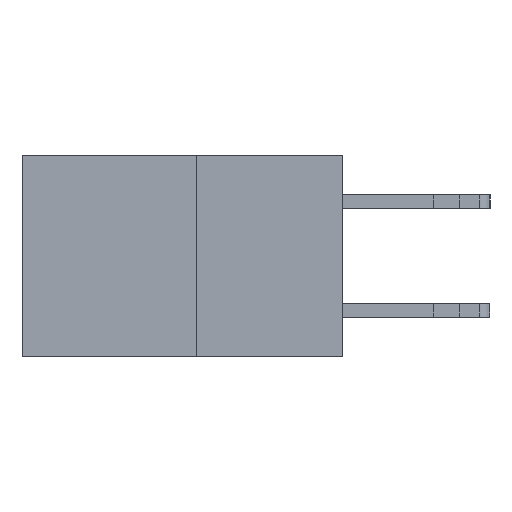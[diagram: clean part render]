
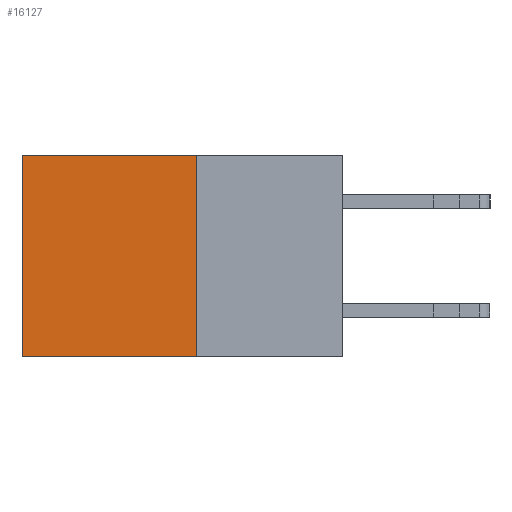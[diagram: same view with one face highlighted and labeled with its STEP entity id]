
A CAD part, left-side view. The second image highlights one B-rep face of the part: STEP entity #16127.
In plain terms, the highlighted planar face has unit normal (-1, 0, 0).
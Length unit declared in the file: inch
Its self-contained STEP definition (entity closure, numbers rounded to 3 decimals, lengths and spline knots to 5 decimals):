
#16 = DIRECTION ( 'NONE',  ( 0., 0., -1. ) ) ;
#331 = CARTESIAN_POINT ( 'NONE',  ( 0.277, 0.27, -0.37 ) ) ;
#516 = LINE ( 'NONE', #19589, #13210 ) ;
#1337 = EDGE_CURVE ( 'NONE', #25789, #11392, #17061, .T. ) ;
#2013 = CARTESIAN_POINT ( 'NONE',  ( 0.277, 0.59, -0.37 ) ) ;
#2298 = FACE_OUTER_BOUND ( 'NONE', #22795, .T. ) ;
#3378 = CARTESIAN_POINT ( 'NONE',  ( 0.277, 0.27, -0.37 ) ) ;
#4542 = DIRECTION ( 'NONE',  ( 0., 0., -1. ) ) ;
#4999 = CARTESIAN_POINT ( 'NONE',  ( 0.277, 0.59, 0. ) ) ;
#5130 = CARTESIAN_POINT ( 'NONE',  ( 0.277, 0.59, -0.37 ) ) ;
#5727 = AXIS2_PLACEMENT_3D ( 'NONE', #3378, #21114, #5905 ) ;
#5905 = DIRECTION ( 'NONE',  ( 0., 0., -1. ) ) ;
#6543 = ORIENTED_EDGE ( 'NONE', *, *, #22734, .F. ) ;
#6626 = ORIENTED_EDGE ( 'NONE', *, *, #10144, .F. ) ;
#7557 = VERTEX_POINT ( 'NONE', #27021 ) ;
#10144 = EDGE_CURVE ( 'NONE', #14666, #11392, #25483, .T. ) ;
#10501 = DIRECTION ( 'NONE',  ( 0., 1., 0. ) ) ;
#11392 = VERTEX_POINT ( 'NONE', #5130 ) ;
#13210 = VECTOR ( 'NONE', #4542, 39.37008 ) ;
#14429 = ORIENTED_EDGE ( 'NONE', *, *, #1337, .T. ) ;
#14666 = VERTEX_POINT ( 'NONE', #20618 ) ;
#15457 = VECTOR ( 'NONE', #16, 39.37008 ) ;
#16127 = ADVANCED_FACE ( 'NONE', ( #2298 ), #18517, .F. ) ;
#17061 = LINE ( 'NONE', #2013, #15457 ) ;
#18300 = EDGE_CURVE ( 'NONE', #7557, #25789, #27808, .T. ) ;
#18517 = PLANE ( 'NONE',  #5727 ) ;
#19589 = CARTESIAN_POINT ( 'NONE',  ( 0.277, 0.27, -0.37 ) ) ;
#20618 = CARTESIAN_POINT ( 'NONE',  ( 0.277, 0.27, -0.37 ) ) ;
#21114 = DIRECTION ( 'NONE',  ( 1., 0., 0. ) ) ;
#21208 = VECTOR ( 'NONE', #22139, 39.37008 ) ;
#22139 = DIRECTION ( 'NONE',  ( 0., 1., 0. ) ) ;
#22734 = EDGE_CURVE ( 'NONE', #7557, #14666, #516, .T. ) ;
#22795 = EDGE_LOOP ( 'NONE', ( #14429, #6626, #6543, #28800 ) ) ;
#25483 = LINE ( 'NONE', #331, #31205 ) ;
#25789 = VERTEX_POINT ( 'NONE', #4999 ) ;
#27021 = CARTESIAN_POINT ( 'NONE',  ( 0.277, 0.27, 0. ) ) ;
#27808 = LINE ( 'NONE', #30190, #21208 ) ;
#28800 = ORIENTED_EDGE ( 'NONE', *, *, #18300, .T. ) ;
#30190 = CARTESIAN_POINT ( 'NONE',  ( 0.277, 0.27, 0. ) ) ;
#31205 = VECTOR ( 'NONE', #10501, 39.37008 ) ;
